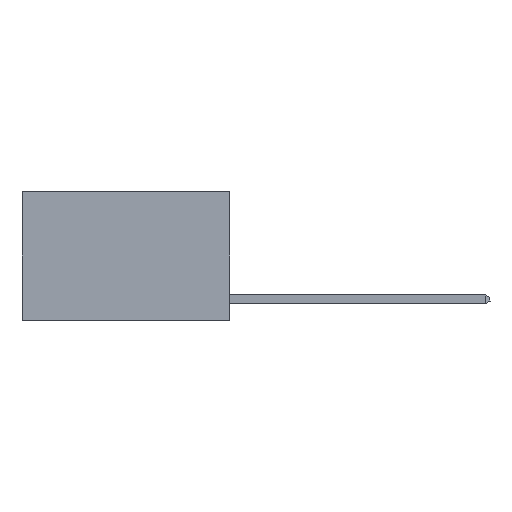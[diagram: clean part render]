
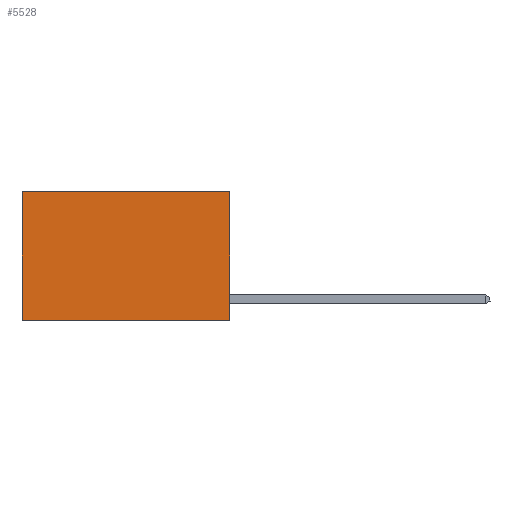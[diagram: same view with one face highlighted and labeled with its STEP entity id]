
A CAD part, left-side view. The second image highlights one B-rep face of the part: STEP entity #5528.
In plain terms, the highlighted planar face has unit normal (-1, 0, 0).
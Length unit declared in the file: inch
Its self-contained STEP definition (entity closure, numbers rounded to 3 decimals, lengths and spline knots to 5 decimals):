
#621 = ORIENTED_EDGE ( 'NONE', *, *, #6932, .T. ) ;
#630 = LINE ( 'NONE', #4084, #1324 ) ;
#901 = VERTEX_POINT ( 'NONE', #8250 ) ;
#902 = CARTESIAN_POINT ( 'NONE',  ( 0.2625, 0., 0. ) ) ;
#1205 = CARTESIAN_POINT ( 'NONE',  ( 0.2625, 0., 0. ) ) ;
#1324 = VECTOR ( 'NONE', #6942, 39.37008 ) ;
#1909 = ORIENTED_EDGE ( 'NONE', *, *, #1955, .F. ) ;
#1955 = EDGE_CURVE ( 'NONE', #7066, #2570, #6985, .T. ) ;
#2148 = VECTOR ( 'NONE', #7738, 39.37008 ) ;
#2570 = VERTEX_POINT ( 'NONE', #4773 ) ;
#3562 = VERTEX_POINT ( 'NONE', #3935 ) ;
#3621 = ORIENTED_EDGE ( 'NONE', *, *, #5984, .T. ) ;
#3739 = AXIS2_PLACEMENT_3D ( 'NONE', #1205, #6296, #9203 ) ;
#3935 = CARTESIAN_POINT ( 'NONE',  ( 0.2625, 0., 0. ) ) ;
#4084 = CARTESIAN_POINT ( 'NONE',  ( 0.2625, 0., 0. ) ) ;
#4377 = ORIENTED_EDGE ( 'NONE', *, *, #5874, .F. ) ;
#4440 = CARTESIAN_POINT ( 'NONE',  ( 0.2625, 0.6, 0. ) ) ;
#4773 = CARTESIAN_POINT ( 'NONE',  ( 0.2625, 0.6, -0.37 ) ) ;
#5455 = PLANE ( 'NONE',  #3739 ) ;
#5528 = ADVANCED_FACE ( 'NONE', ( #6391 ), #5455, .F. ) ;
#5750 = LINE ( 'NONE', #4440, #6534 ) ;
#5874 = EDGE_CURVE ( 'NONE', #3562, #7066, #630, .T. ) ;
#5984 = EDGE_CURVE ( 'NONE', #3562, #901, #6473, .T. ) ;
#6296 = DIRECTION ( 'NONE',  ( 1., 0., 0. ) ) ;
#6391 = FACE_OUTER_BOUND ( 'NONE', #7821, .T. ) ;
#6473 = LINE ( 'NONE', #902, #8228 ) ;
#6534 = VECTOR ( 'NONE', #8918, 39.37008 ) ;
#6932 = EDGE_CURVE ( 'NONE', #901, #2570, #5750, .T. ) ;
#6942 = DIRECTION ( 'NONE',  ( 0., 0., -1. ) ) ;
#6985 = LINE ( 'NONE', #7084, #2148 ) ;
#7066 = VERTEX_POINT ( 'NONE', #9288 ) ;
#7084 = CARTESIAN_POINT ( 'NONE',  ( 0.2625, 0., -0.37 ) ) ;
#7308 = DIRECTION ( 'NONE',  ( 0., 1., 0. ) ) ;
#7738 = DIRECTION ( 'NONE',  ( 0., 1., 0. ) ) ;
#7821 = EDGE_LOOP ( 'NONE', ( #621, #1909, #4377, #3621 ) ) ;
#8228 = VECTOR ( 'NONE', #7308, 39.37008 ) ;
#8250 = CARTESIAN_POINT ( 'NONE',  ( 0.2625, 0.6, 0. ) ) ;
#8918 = DIRECTION ( 'NONE',  ( 0., 0., -1. ) ) ;
#9203 = DIRECTION ( 'NONE',  ( 0., 0., -1. ) ) ;
#9288 = CARTESIAN_POINT ( 'NONE',  ( 0.2625, 0., -0.37 ) ) ;
